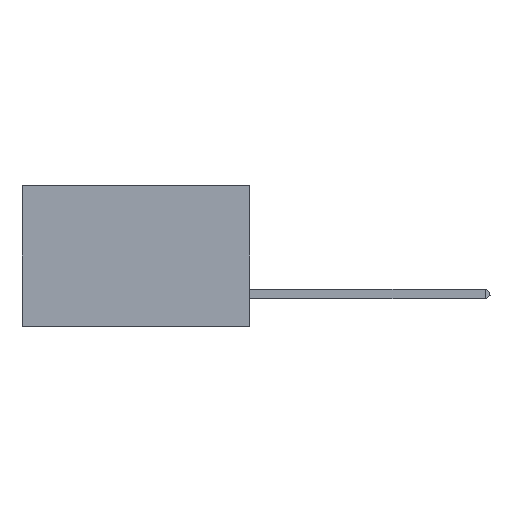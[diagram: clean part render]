
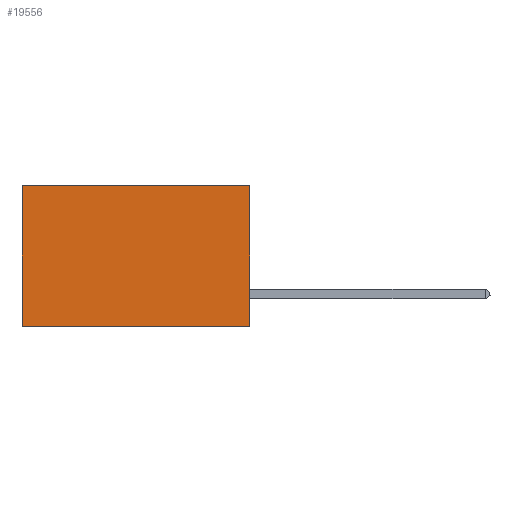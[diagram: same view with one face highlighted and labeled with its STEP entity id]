
A CAD part, left-side view. The second image highlights one B-rep face of the part: STEP entity #19556.
In plain terms, the highlighted planar face has unit normal (-1, 0, 0).
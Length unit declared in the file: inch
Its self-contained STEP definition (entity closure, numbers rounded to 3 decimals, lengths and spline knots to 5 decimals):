
#1268 = ORIENTED_EDGE ( 'NONE', *, *, #2424, .T. ) ;
#1408 = DIRECTION ( 'NONE',  ( 0., 0., -1. ) ) ;
#1665 = CARTESIAN_POINT ( 'NONE',  ( 0.2875, 0., 0. ) ) ;
#1862 = VERTEX_POINT ( 'NONE', #29892 ) ;
#2424 = EDGE_CURVE ( 'NONE', #1862, #34800, #13473, .T. ) ;
#4064 = CARTESIAN_POINT ( 'NONE',  ( 0.2875, 0., -0.37 ) ) ;
#4074 = EDGE_CURVE ( 'NONE', #16538, #1862, #17341, .T. ) ;
#4772 = VECTOR ( 'NONE', #1408, 39.37008 ) ;
#6732 = VECTOR ( 'NONE', #9816, 39.37008 ) ;
#6846 = CARTESIAN_POINT ( 'NONE',  ( 0.2875, 0., 0. ) ) ;
#9816 = DIRECTION ( 'NONE',  ( 0., 0., -1. ) ) ;
#10683 = LINE ( 'NONE', #1665, #6732 ) ;
#11159 = FACE_OUTER_BOUND ( 'NONE', #11383, .T. ) ;
#11383 = EDGE_LOOP ( 'NONE', ( #1268, #12750, #19229, #33661 ) ) ;
#11743 = VERTEX_POINT ( 'NONE', #26432 ) ;
#12750 = ORIENTED_EDGE ( 'NONE', *, *, #16345, .F. ) ;
#13473 = LINE ( 'NONE', #18130, #4772 ) ;
#14714 = VECTOR ( 'NONE', #18202, 39.37008 ) ;
#15305 = LINE ( 'NONE', #4064, #35916 ) ;
#16345 = EDGE_CURVE ( 'NONE', #11743, #34800, #15305, .T. ) ;
#16538 = VERTEX_POINT ( 'NONE', #18212 ) ;
#17341 = LINE ( 'NONE', #6846, #14714 ) ;
#18130 = CARTESIAN_POINT ( 'NONE',  ( 0.2875, 0.6, 0. ) ) ;
#18202 = DIRECTION ( 'NONE',  ( 0., 1., 0. ) ) ;
#18212 = CARTESIAN_POINT ( 'NONE',  ( 0.2875, 0., 0. ) ) ;
#19229 = ORIENTED_EDGE ( 'NONE', *, *, #27622, .F. ) ;
#19556 = ADVANCED_FACE ( 'NONE', ( #11159 ), #21071, .F. ) ;
#20657 = DIRECTION ( 'NONE',  ( 0., 1., 0. ) ) ;
#20951 = CARTESIAN_POINT ( 'NONE',  ( 0.2875, 0., 0. ) ) ;
#21071 = PLANE ( 'NONE',  #32708 ) ;
#26432 = CARTESIAN_POINT ( 'NONE',  ( 0.2875, 0., -0.37 ) ) ;
#26935 = DIRECTION ( 'NONE',  ( 1., 0., 0. ) ) ;
#27622 = EDGE_CURVE ( 'NONE', #16538, #11743, #10683, .T. ) ;
#29052 = CARTESIAN_POINT ( 'NONE',  ( 0.2875, 0.6, -0.37 ) ) ;
#29892 = CARTESIAN_POINT ( 'NONE',  ( 0.2875, 0.6, 0. ) ) ;
#32454 = DIRECTION ( 'NONE',  ( 0., 0., -1. ) ) ;
#32708 = AXIS2_PLACEMENT_3D ( 'NONE', #20951, #26935, #32454 ) ;
#33661 = ORIENTED_EDGE ( 'NONE', *, *, #4074, .T. ) ;
#34800 = VERTEX_POINT ( 'NONE', #29052 ) ;
#35916 = VECTOR ( 'NONE', #20657, 39.37008 ) ;
